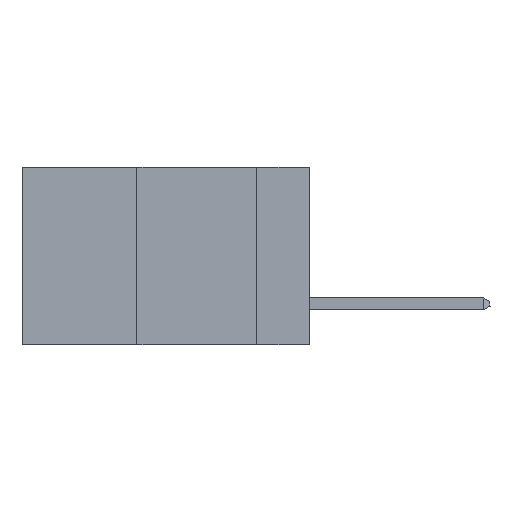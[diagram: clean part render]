
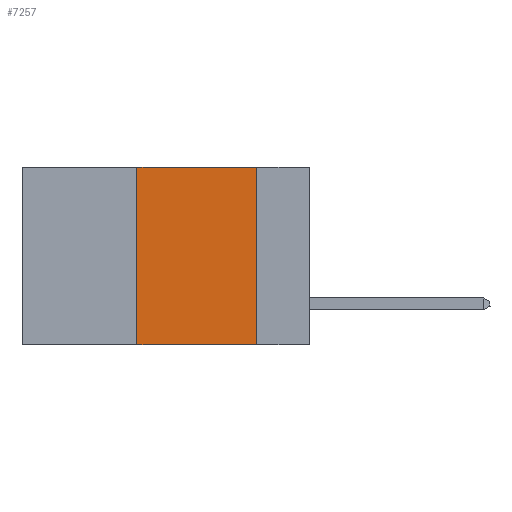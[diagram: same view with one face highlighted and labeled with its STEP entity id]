
A CAD part, left-side view. The second image highlights one B-rep face of the part: STEP entity #7257.
In plain terms, the highlighted planar face has unit normal (-1, 0, 0).
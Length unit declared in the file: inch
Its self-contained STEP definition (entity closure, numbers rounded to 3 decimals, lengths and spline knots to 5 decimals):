
#259 = AXIS2_PLACEMENT_3D ( 'NONE', #4674, #1536, #19406 ) ;
#1165 = VECTOR ( 'NONE', #7618, 39.37008 ) ;
#1536 = DIRECTION ( 'NONE',  ( 1., 0., 0. ) ) ;
#2123 = DIRECTION ( 'NONE',  ( 0., -1., 0. ) ) ;
#2917 = DIRECTION ( 'NONE',  ( 0., 0., -1. ) ) ;
#3463 = VECTOR ( 'NONE', #2917, 39.37008 ) ;
#3710 = VERTEX_POINT ( 'NONE', #8460 ) ;
#4489 = PLANE ( 'NONE',  #259 ) ;
#4616 = LINE ( 'NONE', #13359, #3463 ) ;
#4674 = CARTESIAN_POINT ( 'NONE',  ( 0., 0.6, 0. ) ) ;
#5428 = VERTEX_POINT ( 'NONE', #10784 ) ;
#7257 = ADVANCED_FACE ( 'NONE', ( #7624 ), #4489, .F. ) ;
#7618 = DIRECTION ( 'NONE',  ( 0., -1., 0. ) ) ;
#7624 = FACE_OUTER_BOUND ( 'NONE', #7776, .T. ) ;
#7776 = EDGE_LOOP ( 'NONE', ( #10649, #15422, #17759, #10292 ) ) ;
#8460 = CARTESIAN_POINT ( 'NONE',  ( 0., 0.36, -0.37 ) ) ;
#9680 = EDGE_CURVE ( 'NONE', #3710, #16134, #12212, .T. ) ;
#10292 = ORIENTED_EDGE ( 'NONE', *, *, #9680, .T. ) ;
#10649 = ORIENTED_EDGE ( 'NONE', *, *, #12077, .F. ) ;
#10784 = CARTESIAN_POINT ( 'NONE',  ( 0., 0.11, 0. ) ) ;
#11018 = LINE ( 'NONE', #14145, #13597 ) ;
#11019 = VERTEX_POINT ( 'NONE', #13500 ) ;
#11135 = EDGE_CURVE ( 'NONE', #11019, #5428, #11018, .T. ) ;
#11597 = CARTESIAN_POINT ( 'NONE',  ( 0., 0.36, 0. ) ) ;
#12077 = EDGE_CURVE ( 'NONE', #5428, #16134, #4616, .T. ) ;
#12212 = LINE ( 'NONE', #15034, #1165 ) ;
#12783 = VECTOR ( 'NONE', #14631, 39.37008 ) ;
#13359 = CARTESIAN_POINT ( 'NONE',  ( 0., 0.11, 0. ) ) ;
#13500 = CARTESIAN_POINT ( 'NONE',  ( 0., 0.36, 0. ) ) ;
#13597 = VECTOR ( 'NONE', #2123, 39.37008 ) ;
#14095 = EDGE_CURVE ( 'NONE', #3710, #11019, #16773, .T. ) ;
#14145 = CARTESIAN_POINT ( 'NONE',  ( 0., 0.6, 0. ) ) ;
#14631 = DIRECTION ( 'NONE',  ( 0., 0., 1. ) ) ;
#15034 = CARTESIAN_POINT ( 'NONE',  ( 0., 0.6, -0.37 ) ) ;
#15422 = ORIENTED_EDGE ( 'NONE', *, *, #11135, .F. ) ;
#16134 = VERTEX_POINT ( 'NONE', #18723 ) ;
#16773 = LINE ( 'NONE', #11597, #12783 ) ;
#17759 = ORIENTED_EDGE ( 'NONE', *, *, #14095, .F. ) ;
#18723 = CARTESIAN_POINT ( 'NONE',  ( 0., 0.11, -0.37 ) ) ;
#19406 = DIRECTION ( 'NONE',  ( 0., 0., -1. ) ) ;
